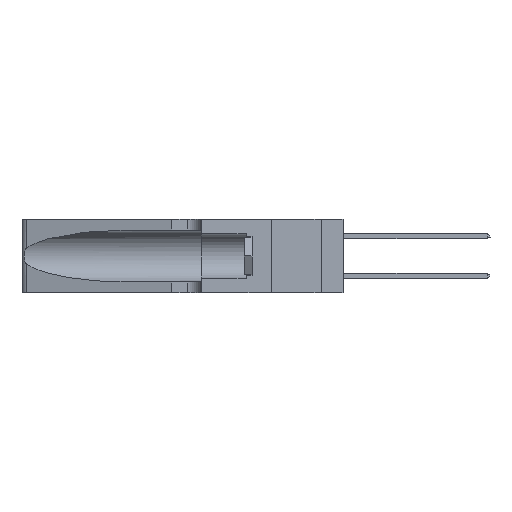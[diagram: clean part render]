
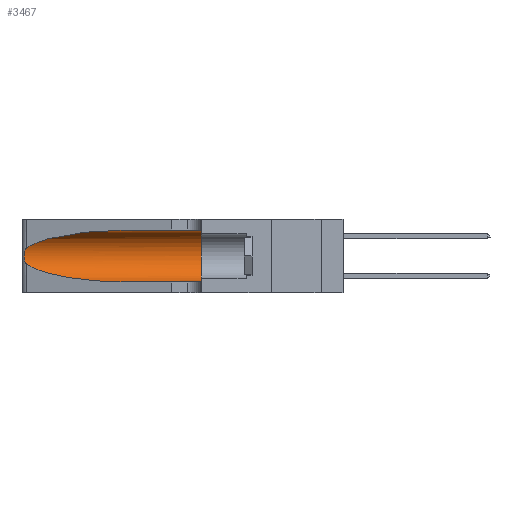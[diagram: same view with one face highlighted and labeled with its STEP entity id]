
A CAD part, left-side view. The second image highlights one B-rep face of the part: STEP entity #3467.
In plain terms, the highlighted cylindrical face has radius 3.308 mm (diameter 6.617 mm), a partial arc.
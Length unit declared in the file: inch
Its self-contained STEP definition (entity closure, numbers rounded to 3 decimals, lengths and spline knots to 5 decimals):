
#788 = DIRECTION ( 'NONE',  ( 0., 0., 1. ) ) ;
#2602 = VERTEX_POINT ( 'NONE', #3200 ) ;
#2991 = CARTESIAN_POINT ( 'NONE',  ( 0.25555, 1.22994, 0.2215 ) ) ;
#3115 =( BOUNDED_CURVE ( )  B_SPLINE_CURVE ( 3, ( #4027, #23189, #15804, #11556 ),
 .UNSPECIFIED., .F., .T. ) 
 B_SPLINE_CURVE_WITH_KNOTS ( ( 4, 4 ),
 ( 3.44316, 4.71239 ),
 .UNSPECIFIED. ) 
 CURVE ( )  GEOMETRIC_REPRESENTATION_ITEM ( )  RATIONAL_B_SPLINE_CURVE ( ( 1., 0.87, 0.87, 1. ) ) 
 REPRESENTATION_ITEM ( '' )  );
#3200 = CARTESIAN_POINT ( 'NONE',  ( 0.1305, 0.72297, 0.05475 ) ) ;
#3467 = ADVANCED_FACE ( 'NONE', ( #28202 ), #37343, .F. ) ;
#4027 = CARTESIAN_POINT ( 'NONE',  ( 0.25487, 1.22718, 0.14631 ) ) ;
#4221 = EDGE_CURVE ( 'NONE', #2602, #24672, #28096, .T. ) ;
#4415 = DIRECTION ( 'NONE',  ( 0., -1., 0. ) ) ;
#5345 = CARTESIAN_POINT ( 'NONE',  ( 0.1305, 0.72297, 0.31525 ) ) ;
#5485 = EDGE_CURVE ( 'NONE', #36428, #13066, #35917, .T. ) ;
#5568 = CARTESIAN_POINT ( 'NONE',  ( 0.18966, 0.96281, 0.31525 ) ) ;
#5901 = CARTESIAN_POINT ( 'NONE',  ( 0.1305, 0.72297, 0.31525 ) ) ;
#6921 = CARTESIAN_POINT ( 'NONE',  ( 0.25555, 1.22993, 0.14849 ) ) ;
#7458 = CARTESIAN_POINT ( 'NONE',  ( 0.25487, 1.22718, 0.22369 ) ) ;
#8178 = EDGE_LOOP ( 'NONE', ( #45458, #48924, #29565, #27915, #37143, #42033 ) ) ;
#10482 = CARTESIAN_POINT ( 'NONE',  ( 0.2373, 1.15595, 0.28018 ) ) ;
#10761 = CARTESIAN_POINT ( 'NONE',  ( 0.25487, 1.22718, 0.14631 ) ) ;
#11556 = CARTESIAN_POINT ( 'NONE',  ( 0.1305, 0.72297, 0.05475 ) ) ;
#11914 = DIRECTION ( 'NONE',  ( 0., -1., 0. ) ) ;
#12512 = AXIS2_PLACEMENT_3D ( 'NONE', #27972, #20626, #788 ) ;
#13066 = VERTEX_POINT ( 'NONE', #13341 ) ;
#13341 = CARTESIAN_POINT ( 'NONE',  ( 0.1305, 0.35, 0.31525 ) ) ;
#13912 = CARTESIAN_POINT ( 'NONE',  ( 0.1305, 0.35, 0.05475 ) ) ;
#14811 = VERTEX_POINT ( 'NONE', #7458 ) ;
#14919 = CARTESIAN_POINT ( 'NONE',  ( 0.25487, 1.22718, 0.14631 ) ) ;
#15259 = CARTESIAN_POINT ( 'NONE',  ( 0.26075, 1.23896, 0.19203 ) ) ;
#15804 = CARTESIAN_POINT ( 'NONE',  ( 0.18966, 0.96281, 0.05475 ) ) ;
#16179 = CARTESIAN_POINT ( 'NONE',  ( 0.1305, 1.61858, 0.05475 ) ) ;
#18684 = CARTESIAN_POINT ( 'NONE',  ( 0.25487, 1.22718, 0.22369 ) ) ;
#20243 = EDGE_CURVE ( 'NONE', #27303, #2602, #3115, .T. ) ;
#20626 = DIRECTION ( 'NONE',  ( 0., 1., 0. ) ) ;
#21405 = VECTOR ( 'NONE', #4415, 39.37008 ) ;
#22489 = CARTESIAN_POINT ( 'NONE',  ( 0.25487, 1.22718, 0.22369 ) ) ;
#23189 = CARTESIAN_POINT ( 'NONE',  ( 0.2373, 1.15595, 0.08982 ) ) ;
#24672 = VERTEX_POINT ( 'NONE', #13912 ) ;
#25045 = B_SPLINE_CURVE_WITH_KNOTS ( 'NONE', 3,
 ( #22489, #2991, #46547, #50511, #30507, #27072, #15259, #26744, #50337, #26394, #42616, #30337, #6921, #14919 ),
 .UNSPECIFIED., .F., .F.,
 ( 4, 2, 2, 2, 2, 2, 4 ),
 ( 0., 0.00027, 0.00053, 0.00107, 0.0016, 0.00187, 0.00214 ),
 .UNSPECIFIED. ) ;
#25544 = VECTOR ( 'NONE', #11914, 39.37008 ) ;
#26394 = CARTESIAN_POINT ( 'NONE',  ( 0.25856, 1.23593, 0.16098 ) ) ;
#26744 = CARTESIAN_POINT ( 'NONE',  ( 0.26075, 1.23896, 0.178 ) ) ;
#26787 = CARTESIAN_POINT ( 'NONE',  ( 0.1305, 1.61858, 0.185 ) ) ;
#27072 = CARTESIAN_POINT ( 'NONE',  ( 0.26018, 1.23835, 0.19895 ) ) ;
#27303 = VERTEX_POINT ( 'NONE', #10761 ) ;
#27915 = ORIENTED_EDGE ( 'NONE', *, *, #4221, .T. ) ;
#27972 = CARTESIAN_POINT ( 'NONE',  ( 0.1305, 0.35, 0.185 ) ) ;
#27982 = CARTESIAN_POINT ( 'NONE',  ( 0.1305, 1.61858, 0.31525 ) ) ;
#28096 = LINE ( 'NONE', #16179, #21405 ) ;
#28202 = FACE_OUTER_BOUND ( 'NONE', #8178, .T. ) ;
#29565 = ORIENTED_EDGE ( 'NONE', *, *, #20243, .T. ) ;
#29757 = CIRCLE ( 'NONE', #12512, 0.13025 ) ;
#30212 = DIRECTION ( 'NONE',  ( 0., -1., 0. ) ) ;
#30337 = CARTESIAN_POINT ( 'NONE',  ( 0.25639, 1.23186, 0.15144 ) ) ;
#30384 =( BOUNDED_CURVE ( )  B_SPLINE_CURVE ( 3, ( #5901, #5568, #10482, #18684 ),
 .UNSPECIFIED., .F., .T. ) 
 B_SPLINE_CURVE_WITH_KNOTS ( ( 4, 4 ),
 ( 1.5708, 2.84003 ),
 .UNSPECIFIED. ) 
 CURVE ( )  GEOMETRIC_REPRESENTATION_ITEM ( )  RATIONAL_B_SPLINE_CURVE ( ( 1., 0.87, 0.87, 1. ) ) 
 REPRESENTATION_ITEM ( '' )  );
#30507 = CARTESIAN_POINT ( 'NONE',  ( 0.25854, 1.2359, 0.20912 ) ) ;
#35917 = LINE ( 'NONE', #27982, #25544 ) ;
#36428 = VERTEX_POINT ( 'NONE', #5345 ) ;
#37143 = ORIENTED_EDGE ( 'NONE', *, *, #37605, .F. ) ;
#37343 = CYLINDRICAL_SURFACE ( 'NONE', #41221, 0.13025 ) ;
#37605 = EDGE_CURVE ( 'NONE', #13066, #24672, #29757, .T. ) ;
#38089 = EDGE_CURVE ( 'NONE', #14811, #27303, #25045, .T. ) ;
#41221 = AXIS2_PLACEMENT_3D ( 'NONE', #26787, #30212, #49866 ) ;
#42033 = ORIENTED_EDGE ( 'NONE', *, *, #5485, .F. ) ;
#42184 = EDGE_CURVE ( 'NONE', #36428, #14811, #30384, .T. ) ;
#42616 = CARTESIAN_POINT ( 'NONE',  ( 0.25789, 1.23486, 0.15765 ) ) ;
#45458 = ORIENTED_EDGE ( 'NONE', *, *, #42184, .T. ) ;
#46547 = CARTESIAN_POINT ( 'NONE',  ( 0.25639, 1.23184, 0.21858 ) ) ;
#48924 = ORIENTED_EDGE ( 'NONE', *, *, #38089, .T. ) ;
#49866 = DIRECTION ( 'NONE',  ( 0., 0., -1. ) ) ;
#50337 = CARTESIAN_POINT ( 'NONE',  ( 0.26017, 1.23833, 0.17102 ) ) ;
#50511 = CARTESIAN_POINT ( 'NONE',  ( 0.25787, 1.23484, 0.2124 ) ) ;
